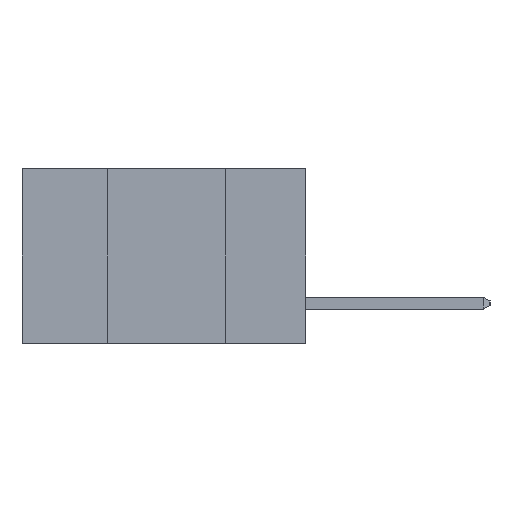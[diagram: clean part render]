
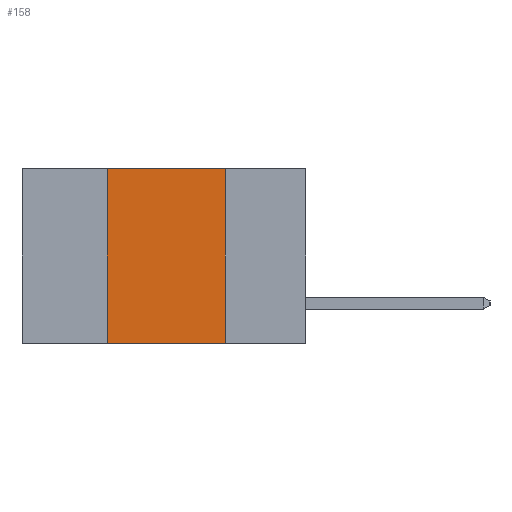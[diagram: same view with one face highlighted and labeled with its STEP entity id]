
A CAD part, left-side view. The second image highlights one B-rep face of the part: STEP entity #158.
In plain terms, the highlighted planar face has unit normal (-1, 0, 0).
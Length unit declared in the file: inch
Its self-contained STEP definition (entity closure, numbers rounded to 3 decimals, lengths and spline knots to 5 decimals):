
#108 = EDGE_LOOP ( 'NONE', ( #9012, #8453, #11386, #8959 ) ) ;
#158 = ADVANCED_FACE ( 'NONE', ( #4051 ), #4150, .F. ) ;
#773 = VECTOR ( 'NONE', #15375, 39.37008 ) ;
#936 = VERTEX_POINT ( 'NONE', #5976 ) ;
#1030 = VERTEX_POINT ( 'NONE', #7400 ) ;
#2550 = EDGE_CURVE ( 'NONE', #5435, #936, #13913, .T. ) ;
#2669 = LINE ( 'NONE', #11497, #5642 ) ;
#3035 = VECTOR ( 'NONE', #4709, 39.37008 ) ;
#3296 = CARTESIAN_POINT ( 'NONE',  ( 0., 0.17, -0.37 ) ) ;
#3885 = CARTESIAN_POINT ( 'NONE',  ( 0., 0.42, 0. ) ) ;
#4051 = FACE_OUTER_BOUND ( 'NONE', #108, .T. ) ;
#4150 = PLANE ( 'NONE',  #4159 ) ;
#4159 = AXIS2_PLACEMENT_3D ( 'NONE', #8553, #8609, #13206 ) ;
#4709 = DIRECTION ( 'NONE',  ( 0., -1., 0. ) ) ;
#5393 = CARTESIAN_POINT ( 'NONE',  ( 0., 0.6, 0. ) ) ;
#5422 = DIRECTION ( 'NONE',  ( 0., 0., -1. ) ) ;
#5435 = VERTEX_POINT ( 'NONE', #12692 ) ;
#5642 = VECTOR ( 'NONE', #5422, 39.37008 ) ;
#5976 = CARTESIAN_POINT ( 'NONE',  ( 0., 0.17, 0. ) ) ;
#6435 = LINE ( 'NONE', #13219, #3035 ) ;
#7361 = VECTOR ( 'NONE', #12499, 39.37008 ) ;
#7400 = CARTESIAN_POINT ( 'NONE',  ( 0., 0.42, -0.37 ) ) ;
#7740 = LINE ( 'NONE', #3885, #7361 ) ;
#8453 = ORIENTED_EDGE ( 'NONE', *, *, #2550, .F. ) ;
#8553 = CARTESIAN_POINT ( 'NONE',  ( 0., 0.6, 0. ) ) ;
#8609 = DIRECTION ( 'NONE',  ( 1., 0., 0. ) ) ;
#8959 = ORIENTED_EDGE ( 'NONE', *, *, #15304, .T. ) ;
#9012 = ORIENTED_EDGE ( 'NONE', *, *, #9663, .F. ) ;
#9663 = EDGE_CURVE ( 'NONE', #936, #13979, #2669, .T. ) ;
#11386 = ORIENTED_EDGE ( 'NONE', *, *, #12861, .F. ) ;
#11497 = CARTESIAN_POINT ( 'NONE',  ( 0., 0.17, 0. ) ) ;
#12499 = DIRECTION ( 'NONE',  ( 0., 0., 1. ) ) ;
#12692 = CARTESIAN_POINT ( 'NONE',  ( 0., 0.42, 0. ) ) ;
#12861 = EDGE_CURVE ( 'NONE', #1030, #5435, #7740, .T. ) ;
#13206 = DIRECTION ( 'NONE',  ( 0., 0., -1. ) ) ;
#13219 = CARTESIAN_POINT ( 'NONE',  ( 0., 0.6, -0.37 ) ) ;
#13913 = LINE ( 'NONE', #5393, #773 ) ;
#13979 = VERTEX_POINT ( 'NONE', #3296 ) ;
#15304 = EDGE_CURVE ( 'NONE', #1030, #13979, #6435, .T. ) ;
#15375 = DIRECTION ( 'NONE',  ( 0., -1., 0. ) ) ;
